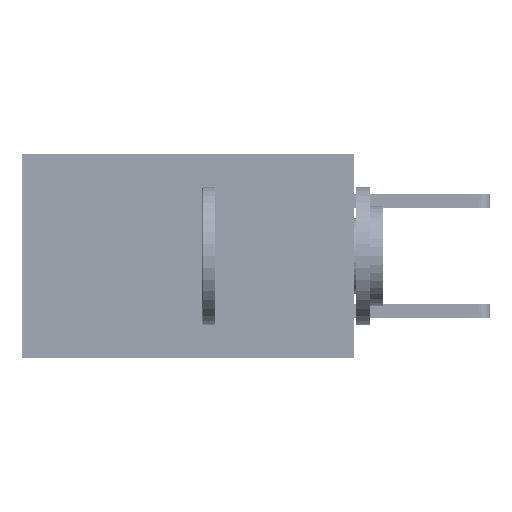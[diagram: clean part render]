
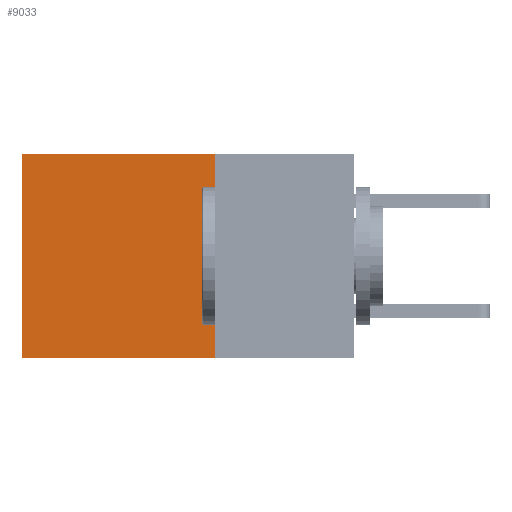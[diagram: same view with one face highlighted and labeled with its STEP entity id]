
A CAD part, left-side view. The second image highlights one B-rep face of the part: STEP entity #9033.
In plain terms, the highlighted planar face has unit normal (-1, 0, 0).
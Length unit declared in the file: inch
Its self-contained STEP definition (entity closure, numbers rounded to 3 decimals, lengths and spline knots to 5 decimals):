
#204 = ORIENTED_EDGE ( 'NONE', *, *, #28992, .F. ) ;
#903 = DIRECTION ( 'NONE',  ( 0., 1., 0. ) ) ;
#1454 = LINE ( 'NONE', #17182, #36023 ) ;
#4529 = CARTESIAN_POINT ( 'NONE',  ( 0.2875, 0.6, 0. ) ) ;
#4907 = LINE ( 'NONE', #23290, #18358 ) ;
#6101 = VECTOR ( 'NONE', #38945, 39.37008 ) ;
#6111 = VERTEX_POINT ( 'NONE', #18547 ) ;
#6279 = EDGE_LOOP ( 'NONE', ( #25567, #204, #10502, #16527 ) ) ;
#7135 = DIRECTION ( 'NONE',  ( 0., 0., -1. ) ) ;
#7437 = EDGE_CURVE ( 'NONE', #28973, #41393, #31866, .T. ) ;
#9033 = ADVANCED_FACE ( 'NONE', ( #22351 ), #37613, .F. ) ;
#10502 = ORIENTED_EDGE ( 'NONE', *, *, #18841, .F. ) ;
#15128 = CARTESIAN_POINT ( 'NONE',  ( 0.2875, 0.25, 0. ) ) ;
#15287 = DIRECTION ( 'NONE',  ( 1., 0., 0. ) ) ;
#16002 = DIRECTION ( 'NONE',  ( 0., 1., 0. ) ) ;
#16527 = ORIENTED_EDGE ( 'NONE', *, *, #30156, .T. ) ;
#17182 = CARTESIAN_POINT ( 'NONE',  ( 0.2875, 0.25, 0. ) ) ;
#18358 = VECTOR ( 'NONE', #903, 39.37008 ) ;
#18547 = CARTESIAN_POINT ( 'NONE',  ( 0.2875, 0.25, -0.37 ) ) ;
#18841 = EDGE_CURVE ( 'NONE', #38791, #6111, #1454, .T. ) ;
#22351 = FACE_OUTER_BOUND ( 'NONE', #6279, .T. ) ;
#23290 = CARTESIAN_POINT ( 'NONE',  ( 0.2875, 0.25, 0. ) ) ;
#23390 = CARTESIAN_POINT ( 'NONE',  ( 0.2875, 0.25, -0.37 ) ) ;
#25567 = ORIENTED_EDGE ( 'NONE', *, *, #7437, .T. ) ;
#28973 = VERTEX_POINT ( 'NONE', #42135 ) ;
#28992 = EDGE_CURVE ( 'NONE', #6111, #41393, #46023, .T. ) ;
#30156 = EDGE_CURVE ( 'NONE', #38791, #28973, #4907, .T. ) ;
#31866 = LINE ( 'NONE', #4529, #6101 ) ;
#32602 = CARTESIAN_POINT ( 'NONE',  ( 0.2875, 0.25, 0. ) ) ;
#36023 = VECTOR ( 'NONE', #39664, 39.37008 ) ;
#37613 = PLANE ( 'NONE',  #48314 ) ;
#38791 = VERTEX_POINT ( 'NONE', #32602 ) ;
#38945 = DIRECTION ( 'NONE',  ( 0., 0., -1. ) ) ;
#39664 = DIRECTION ( 'NONE',  ( 0., 0., -1. ) ) ;
#41393 = VERTEX_POINT ( 'NONE', #47806 ) ;
#42135 = CARTESIAN_POINT ( 'NONE',  ( 0.2875, 0.6, 0. ) ) ;
#46023 = LINE ( 'NONE', #23390, #48347 ) ;
#47806 = CARTESIAN_POINT ( 'NONE',  ( 0.2875, 0.6, -0.37 ) ) ;
#48314 = AXIS2_PLACEMENT_3D ( 'NONE', #15128, #15287, #7135 ) ;
#48347 = VECTOR ( 'NONE', #16002, 39.37008 ) ;
